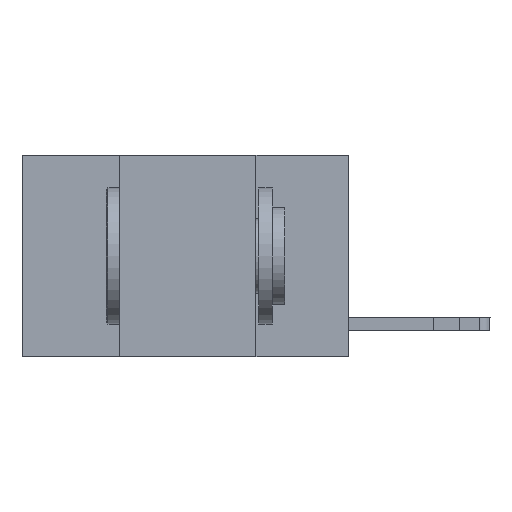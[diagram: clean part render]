
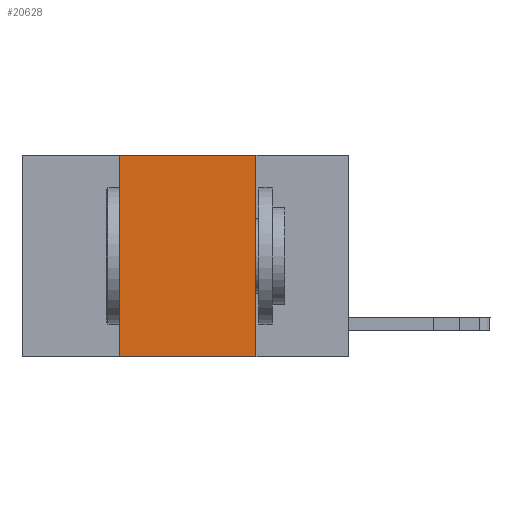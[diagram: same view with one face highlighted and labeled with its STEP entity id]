
A CAD part, left-side view. The second image highlights one B-rep face of the part: STEP entity #20628.
In plain terms, the highlighted planar face has unit normal (-1, 0, 0).
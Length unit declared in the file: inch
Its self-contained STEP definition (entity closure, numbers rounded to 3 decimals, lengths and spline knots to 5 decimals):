
#879 = CARTESIAN_POINT ( 'NONE',  ( 0., 0.6, 0. ) ) ;
#884 = CARTESIAN_POINT ( 'NONE',  ( 0., 0.6, 0. ) ) ;
#2477 = ORIENTED_EDGE ( 'NONE', *, *, #15238, .F. ) ;
#2685 = DIRECTION ( 'NONE',  ( 0., 0., -1. ) ) ;
#2992 = DIRECTION ( 'NONE',  ( 0., -1., 0. ) ) ;
#3521 = LINE ( 'NONE', #14850, #4175 ) ;
#3790 = VERTEX_POINT ( 'NONE', #14130 ) ;
#4175 = VECTOR ( 'NONE', #2685, 39.37008 ) ;
#5051 = DIRECTION ( 'NONE',  ( 1., 0., 0. ) ) ;
#5988 = VECTOR ( 'NONE', #13231, 39.37008 ) ;
#7762 = LINE ( 'NONE', #23589, #17916 ) ;
#8103 = FACE_OUTER_BOUND ( 'NONE', #17183, .T. ) ;
#8278 = EDGE_CURVE ( 'NONE', #3790, #23938, #7762, .T. ) ;
#8625 = CARTESIAN_POINT ( 'NONE',  ( 0., 0.17, 0. ) ) ;
#8802 = VERTEX_POINT ( 'NONE', #13066 ) ;
#9360 = CARTESIAN_POINT ( 'NONE',  ( 0., 0.17, -0.37 ) ) ;
#11653 = EDGE_CURVE ( 'NONE', #3790, #8802, #12046, .T. ) ;
#12046 = LINE ( 'NONE', #21292, #5988 ) ;
#13066 = CARTESIAN_POINT ( 'NONE',  ( 0., 0.42, 0. ) ) ;
#13231 = DIRECTION ( 'NONE',  ( 0., 0., 1. ) ) ;
#14130 = CARTESIAN_POINT ( 'NONE',  ( 0., 0.42, -0.37 ) ) ;
#14552 = ORIENTED_EDGE ( 'NONE', *, *, #25053, .F. ) ;
#14850 = CARTESIAN_POINT ( 'NONE',  ( 0., 0.17, 0. ) ) ;
#15238 = EDGE_CURVE ( 'NONE', #17530, #23938, #3521, .T. ) ;
#15829 = ORIENTED_EDGE ( 'NONE', *, *, #8278, .T. ) ;
#17183 = EDGE_LOOP ( 'NONE', ( #2477, #14552, #25307, #15829 ) ) ;
#17315 = AXIS2_PLACEMENT_3D ( 'NONE', #879, #5051, #19227 ) ;
#17530 = VERTEX_POINT ( 'NONE', #8625 ) ;
#17916 = VECTOR ( 'NONE', #25611, 39.37008 ) ;
#19227 = DIRECTION ( 'NONE',  ( 0., 0., -1. ) ) ;
#20115 = VECTOR ( 'NONE', #2992, 39.37008 ) ;
#20628 = ADVANCED_FACE ( 'NONE', ( #8103 ), #25201, .F. ) ;
#21292 = CARTESIAN_POINT ( 'NONE',  ( 0., 0.42, 0. ) ) ;
#23589 = CARTESIAN_POINT ( 'NONE',  ( 0., 0.6, -0.37 ) ) ;
#23938 = VERTEX_POINT ( 'NONE', #9360 ) ;
#25053 = EDGE_CURVE ( 'NONE', #8802, #17530, #26099, .T. ) ;
#25201 = PLANE ( 'NONE',  #17315 ) ;
#25307 = ORIENTED_EDGE ( 'NONE', *, *, #11653, .F. ) ;
#25611 = DIRECTION ( 'NONE',  ( 0., -1., 0. ) ) ;
#26099 = LINE ( 'NONE', #884, #20115 ) ;
